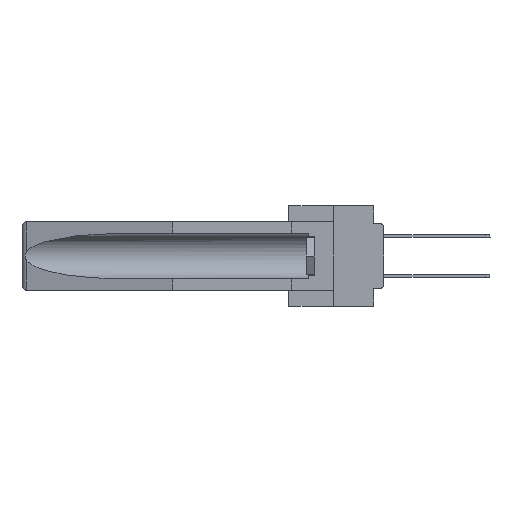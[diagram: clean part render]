
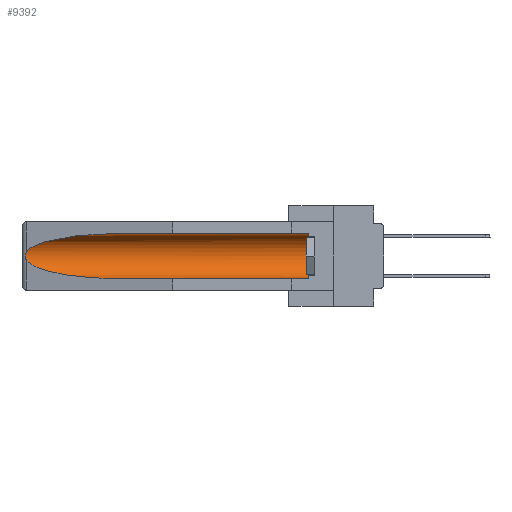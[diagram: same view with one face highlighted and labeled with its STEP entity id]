
A CAD part, left-side view. The second image highlights one B-rep face of the part: STEP entity #9392.
In plain terms, the highlighted cylindrical face has radius 2.857 mm (diameter 5.715 mm), a partial arc.
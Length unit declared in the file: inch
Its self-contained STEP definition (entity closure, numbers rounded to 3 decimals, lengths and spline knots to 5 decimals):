
#285 = CARTESIAN_POINT ( 'NONE',  ( 0.155, 1.07973, -0.284 ) ) ;
#394 = EDGE_CURVE ( 'NONE', #22247, #30145, #18685, .T. ) ;
#482 = CARTESIAN_POINT ( 'NONE',  ( 0.21114, 1.30732, -0.284 ) ) ;
#1305 = CARTESIAN_POINT ( 'NONE',  ( 0.26537, 1.52718, -0.14972 ) ) ;
#1824 = CARTESIAN_POINT ( 'NONE',  ( 0.26655, 1.53094, -0.18657 ) ) ;
#2040 = LINE ( 'NONE', #29679, #9302 ) ;
#2554 = ORIENTED_EDGE ( 'NONE', *, *, #394, .T. ) ;
#4214 = CIRCLE ( 'NONE', #7603, 0.1125 ) ;
#6383 = ORIENTED_EDGE ( 'NONE', *, *, #28575, .T. ) ;
#6423 = LINE ( 'NONE', #8913, #8521 ) ;
#7603 = AXIS2_PLACEMENT_3D ( 'NONE', #28548, #31738, #28196 ) ;
#7885 = ORIENTED_EDGE ( 'NONE', *, *, #24956, .F. ) ;
#8521 = VECTOR ( 'NONE', #33516, 39.37008 ) ;
#8913 = CARTESIAN_POINT ( 'NONE',  ( 0.155, -0.30754, -0.284 ) ) ;
#9302 = VECTOR ( 'NONE', #16106, 39.37008 ) ;
#9392 = ADVANCED_FACE ( 'NONE', ( #17295 ), #20155, .F. ) ;
#9814 = VERTEX_POINT ( 'NONE', #28317 ) ;
#10161 = CARTESIAN_POINT ( 'NONE',  ( 0.155, 0.126, -0.284 ) ) ;
#12164 = EDGE_CURVE ( 'NONE', #28852, #24439, #22346, .T. ) ;
#12662 = CARTESIAN_POINT ( 'NONE',  ( 0.2673, 1.53269, -0.17917 ) ) ;
#12832 = CARTESIAN_POINT ( 'NONE',  ( 0.26537, 1.52718, -0.19328 ) ) ;
#13493 = ORIENTED_EDGE ( 'NONE', *, *, #21819, .T. ) ;
#14729 = ORIENTED_EDGE ( 'NONE', *, *, #31670, .T. ) ;
#15337 = CARTESIAN_POINT ( 'NONE',  ( 0.26597, 1.52961, -0.15275 ) ) ;
#16106 = DIRECTION ( 'NONE',  ( 0., 1., 0. ) ) ;
#16825 = CARTESIAN_POINT ( 'NONE',  ( 0.25451, 1.48313, -0.09465 ) ) ;
#17295 = FACE_OUTER_BOUND ( 'NONE', #21889, .T. ) ;
#18685 =( BOUNDED_CURVE ( )  B_SPLINE_CURVE ( 3, ( #22187, #30405, #16825, #27715 ),
 .UNSPECIFIED., .F., .F. ) 
 B_SPLINE_CURVE_WITH_KNOTS ( ( 4, 4 ),
 ( 4.71239, 6.08839 ),
 .UNSPECIFIED. ) 
 CURVE ( )  GEOMETRIC_REPRESENTATION_ITEM ( )  RATIONAL_B_SPLINE_CURVE ( ( 1., 0.848, 0.848, 1. ) ) 
 REPRESENTATION_ITEM ( '' )  );
#19071 = ORIENTED_EDGE ( 'NONE', *, *, #12164, .T. ) ;
#19699 = CARTESIAN_POINT ( 'NONE',  ( 0.26537, 1.52718, -0.14972 ) ) ;
#20155 = CYLINDRICAL_SURFACE ( 'NONE', #21069, 0.1125 ) ;
#20695 = CARTESIAN_POINT ( 'NONE',  ( 0.2673, 1.5327, -0.16383 ) ) ;
#21069 = AXIS2_PLACEMENT_3D ( 'NONE', #33190, #23020, #33858 ) ;
#21819 = EDGE_CURVE ( 'NONE', #30145, #28852, #34506, .T. ) ;
#21834 = VERTEX_POINT ( 'NONE', #10161 ) ;
#21889 = EDGE_LOOP ( 'NONE', ( #2554, #13493, #19071, #7885, #14729, #6383 ) ) ;
#22187 = CARTESIAN_POINT ( 'NONE',  ( 0.155, 1.07973, -0.059 ) ) ;
#22214 = CARTESIAN_POINT ( 'NONE',  ( 0.155, 1.07973, -0.284 ) ) ;
#22247 = VERTEX_POINT ( 'NONE', #33669 ) ;
#22346 =( BOUNDED_CURVE ( )  B_SPLINE_CURVE ( 3, ( #33256, #30947, #482, #22214 ),
 .UNSPECIFIED., .F., .F. ) 
 B_SPLINE_CURVE_WITH_KNOTS ( ( 4, 4 ),
 ( 0.1948, 1.5708 ),
 .UNSPECIFIED. ) 
 CURVE ( )  GEOMETRIC_REPRESENTATION_ITEM ( )  RATIONAL_B_SPLINE_CURVE ( ( 1., 0.848, 0.848, 1. ) ) 
 REPRESENTATION_ITEM ( '' )  );
#23020 = DIRECTION ( 'NONE',  ( 0., 1., 0. ) ) ;
#23033 = CARTESIAN_POINT ( 'NONE',  ( 0.26654, 1.53092, -0.15636 ) ) ;
#24439 = VERTEX_POINT ( 'NONE', #285 ) ;
#24956 = EDGE_CURVE ( 'NONE', #21834, #24439, #6423, .T. ) ;
#25720 = CARTESIAN_POINT ( 'NONE',  ( 0.26537, 1.52718, -0.19328 ) ) ;
#26241 = CARTESIAN_POINT ( 'NONE',  ( 0.2675, 1.53308, -0.17534 ) ) ;
#27715 = CARTESIAN_POINT ( 'NONE',  ( 0.26537, 1.52718, -0.14972 ) ) ;
#28196 = DIRECTION ( 'NONE',  ( 0., 0., 1. ) ) ;
#28317 = CARTESIAN_POINT ( 'NONE',  ( 0.155, 0.126, -0.059 ) ) ;
#28548 = CARTESIAN_POINT ( 'NONE',  ( 0.155, 0.126, -0.1715 ) ) ;
#28575 = EDGE_CURVE ( 'NONE', #9814, #22247, #2040, .T. ) ;
#28852 = VERTEX_POINT ( 'NONE', #25720 ) ;
#29679 = CARTESIAN_POINT ( 'NONE',  ( 0.155, -0.30754, -0.059 ) ) ;
#30145 = VERTEX_POINT ( 'NONE', #19699 ) ;
#30405 = CARTESIAN_POINT ( 'NONE',  ( 0.21114, 1.30732, -0.059 ) ) ;
#30947 = CARTESIAN_POINT ( 'NONE',  ( 0.25451, 1.48313, -0.24835 ) ) ;
#31583 = CARTESIAN_POINT ( 'NONE',  ( 0.2675, 1.53308, -0.16763 ) ) ;
#31670 = EDGE_CURVE ( 'NONE', #21834, #9814, #4214, .T. ) ;
#31738 = DIRECTION ( 'NONE',  ( 0., -1., 0. ) ) ;
#33190 = CARTESIAN_POINT ( 'NONE',  ( 0.155, -0.30754, -0.1715 ) ) ;
#33256 = CARTESIAN_POINT ( 'NONE',  ( 0.26537, 1.52718, -0.19328 ) ) ;
#33516 = DIRECTION ( 'NONE',  ( 0., 1., 0. ) ) ;
#33535 = CARTESIAN_POINT ( 'NONE',  ( 0.26597, 1.5296, -0.19026 ) ) ;
#33669 = CARTESIAN_POINT ( 'NONE',  ( 0.155, 1.07973, -0.059 ) ) ;
#33858 = DIRECTION ( 'NONE',  ( 0., 0., 1. ) ) ;
#34506 = B_SPLINE_CURVE_WITH_KNOTS ( 'NONE', 3,
 ( #1305, #15337, #23033, #20695, #31583, #26241, #12662, #1824, #33535, #12832 ),
 .UNSPECIFIED., .F., .F.,
 ( 4, 2, 2, 2, 4 ),
 ( 0., 0.00029, 0.00058, 0.00087, 0.00117 ),
 .UNSPECIFIED. ) ;
